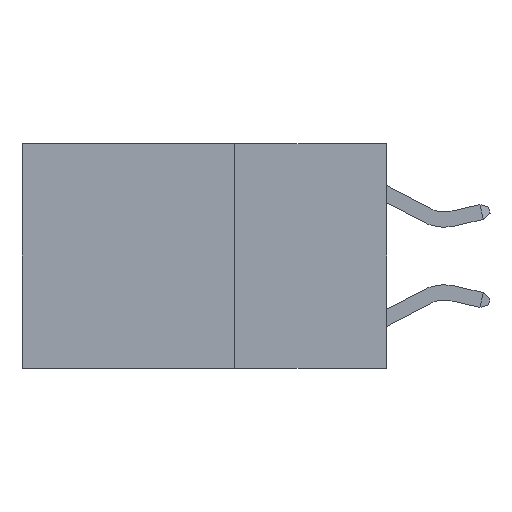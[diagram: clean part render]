
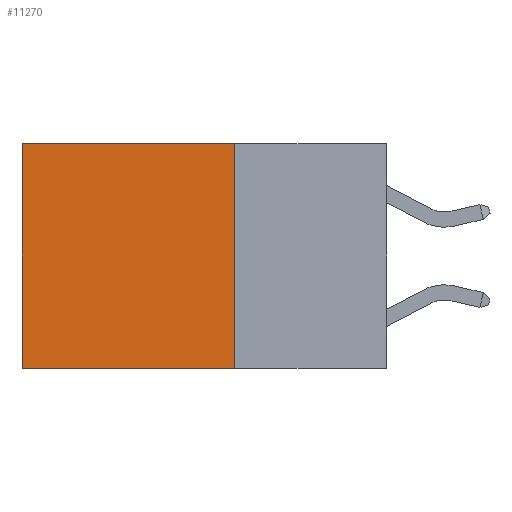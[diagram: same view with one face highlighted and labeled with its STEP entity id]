
A CAD part, left-side view. The second image highlights one B-rep face of the part: STEP entity #11270.
In plain terms, the highlighted planar face has unit normal (-1, 0, 0).
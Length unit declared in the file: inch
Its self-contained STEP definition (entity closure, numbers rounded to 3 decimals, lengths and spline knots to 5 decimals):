
#225 = VECTOR ( 'NONE', #10477, 39.37008 ) ;
#379 = PLANE ( 'NONE',  #11229 ) ;
#958 = ORIENTED_EDGE ( 'NONE', *, *, #2395, .F. ) ;
#1069 = VERTEX_POINT ( 'NONE', #9706 ) ;
#1590 = VERTEX_POINT ( 'NONE', #6764 ) ;
#1661 = CARTESIAN_POINT ( 'NONE',  ( 0.2625, 0.25, 0. ) ) ;
#2395 = EDGE_CURVE ( 'NONE', #13664, #1590, #10266, .T. ) ;
#2739 = VECTOR ( 'NONE', #5984, 39.37008 ) ;
#3759 = FACE_OUTER_BOUND ( 'NONE', #11977, .T. ) ;
#4351 = DIRECTION ( 'NONE',  ( 0., 0., -1. ) ) ;
#4494 = VERTEX_POINT ( 'NONE', #11283 ) ;
#5117 = CARTESIAN_POINT ( 'NONE',  ( 0.2625, 0.25, -0.37 ) ) ;
#5259 = ORIENTED_EDGE ( 'NONE', *, *, #15323, .F. ) ;
#5429 = VECTOR ( 'NONE', #8260, 39.37008 ) ;
#5984 = DIRECTION ( 'NONE',  ( 0., 1., 0. ) ) ;
#6162 = LINE ( 'NONE', #14597, #2739 ) ;
#6764 = CARTESIAN_POINT ( 'NONE',  ( 0.2625, 0.6, -0.37 ) ) ;
#7009 = VECTOR ( 'NONE', #11492, 39.37008 ) ;
#8260 = DIRECTION ( 'NONE',  ( 0., 0., -1. ) ) ;
#8690 = EDGE_CURVE ( 'NONE', #4494, #1069, #6162, .T. ) ;
#8888 = ORIENTED_EDGE ( 'NONE', *, *, #8690, .T. ) ;
#9674 = EDGE_CURVE ( 'NONE', #1069, #1590, #13636, .T. ) ;
#9706 = CARTESIAN_POINT ( 'NONE',  ( 0.2625, 0.6, 0. ) ) ;
#10266 = LINE ( 'NONE', #10995, #7009 ) ;
#10477 = DIRECTION ( 'NONE',  ( 0., 0., -1. ) ) ;
#10995 = CARTESIAN_POINT ( 'NONE',  ( 0.2625, 0.25, -0.37 ) ) ;
#11229 = AXIS2_PLACEMENT_3D ( 'NONE', #1661, #11759, #4351 ) ;
#11270 = ADVANCED_FACE ( 'NONE', ( #3759 ), #379, .F. ) ;
#11283 = CARTESIAN_POINT ( 'NONE',  ( 0.2625, 0.25, 0. ) ) ;
#11492 = DIRECTION ( 'NONE',  ( 0., 1., 0. ) ) ;
#11759 = DIRECTION ( 'NONE',  ( 1., 0., 0. ) ) ;
#11977 = EDGE_LOOP ( 'NONE', ( #15202, #958, #5259, #8888 ) ) ;
#12837 = CARTESIAN_POINT ( 'NONE',  ( 0.2625, 0.6, 0. ) ) ;
#13636 = LINE ( 'NONE', #12837, #225 ) ;
#13664 = VERTEX_POINT ( 'NONE', #5117 ) ;
#14390 = CARTESIAN_POINT ( 'NONE',  ( 0.2625, 0.25, 0. ) ) ;
#14597 = CARTESIAN_POINT ( 'NONE',  ( 0.2625, 0.25, 0. ) ) ;
#15202 = ORIENTED_EDGE ( 'NONE', *, *, #9674, .T. ) ;
#15323 = EDGE_CURVE ( 'NONE', #4494, #13664, #15625, .T. ) ;
#15625 = LINE ( 'NONE', #14390, #5429 ) ;
